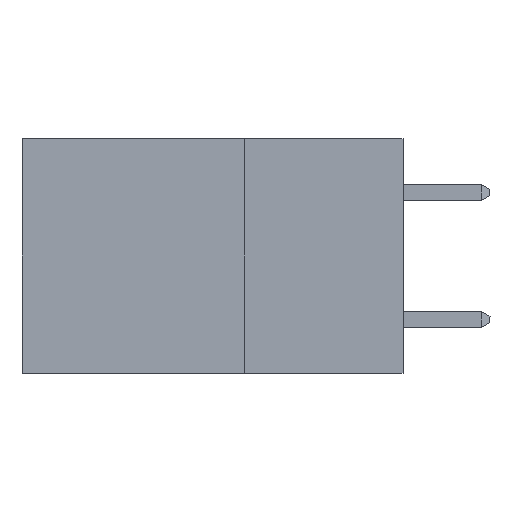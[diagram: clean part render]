
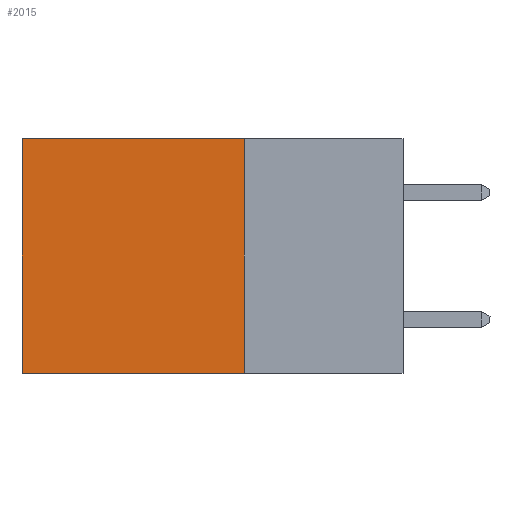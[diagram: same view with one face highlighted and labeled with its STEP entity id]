
A CAD part, left-side view. The second image highlights one B-rep face of the part: STEP entity #2015.
In plain terms, the highlighted planar face has unit normal (-1, 0, 0).
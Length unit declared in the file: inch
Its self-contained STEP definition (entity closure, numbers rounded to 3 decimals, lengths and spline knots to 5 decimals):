
#358 = VERTEX_POINT ( 'NONE', #6611 ) ;
#399 = AXIS2_PLACEMENT_3D ( 'NONE', #697, #4720, #6745 ) ;
#561 = VERTEX_POINT ( 'NONE', #2709 ) ;
#697 = CARTESIAN_POINT ( 'NONE',  ( 0.2875, 0.25, 0. ) ) ;
#1457 = LINE ( 'NONE', #3317, #11266 ) ;
#1633 = EDGE_CURVE ( 'NONE', #4223, #561, #1994, .T. ) ;
#1644 = PLANE ( 'NONE',  #399 ) ;
#1994 = LINE ( 'NONE', #8250, #9449 ) ;
#2015 = ADVANCED_FACE ( 'NONE', ( #6815 ), #1644, .F. ) ;
#2630 = DIRECTION ( 'NONE',  ( 0., 0., -1. ) ) ;
#2709 = CARTESIAN_POINT ( 'NONE',  ( 0.2875, 0.6, -0.37 ) ) ;
#2803 = CARTESIAN_POINT ( 'NONE',  ( 0.2875, 0.25, -0.37 ) ) ;
#2995 = EDGE_CURVE ( 'NONE', #3284, #358, #5194, .T. ) ;
#3284 = VERTEX_POINT ( 'NONE', #6817 ) ;
#3317 = CARTESIAN_POINT ( 'NONE',  ( 0.2875, 0.25, 0. ) ) ;
#3646 = LINE ( 'NONE', #8833, #11497 ) ;
#4223 = VERTEX_POINT ( 'NONE', #2803 ) ;
#4720 = DIRECTION ( 'NONE',  ( 1., 0., 0. ) ) ;
#5014 = ORIENTED_EDGE ( 'NONE', *, *, #5019, .T. ) ;
#5019 = EDGE_CURVE ( 'NONE', #358, #561, #3646, .T. ) ;
#5194 = LINE ( 'NONE', #6267, #9947 ) ;
#5873 = EDGE_CURVE ( 'NONE', #3284, #4223, #1457, .T. ) ;
#6267 = CARTESIAN_POINT ( 'NONE',  ( 0.2875, 0.25, 0. ) ) ;
#6611 = CARTESIAN_POINT ( 'NONE',  ( 0.2875, 0.6, 0. ) ) ;
#6745 = DIRECTION ( 'NONE',  ( 0., 0., -1. ) ) ;
#6815 = FACE_OUTER_BOUND ( 'NONE', #11611, .T. ) ;
#6817 = CARTESIAN_POINT ( 'NONE',  ( 0.2875, 0.25, 0. ) ) ;
#7578 = ORIENTED_EDGE ( 'NONE', *, *, #1633, .F. ) ;
#8250 = CARTESIAN_POINT ( 'NONE',  ( 0.2875, 0.25, -0.37 ) ) ;
#8833 = CARTESIAN_POINT ( 'NONE',  ( 0.2875, 0.6, 0. ) ) ;
#9449 = VECTOR ( 'NONE', #12331, 39.37008 ) ;
#9947 = VECTOR ( 'NONE', #11298, 39.37008 ) ;
#10048 = ORIENTED_EDGE ( 'NONE', *, *, #2995, .T. ) ;
#11266 = VECTOR ( 'NONE', #12665, 39.37008 ) ;
#11298 = DIRECTION ( 'NONE',  ( 0., 1., 0. ) ) ;
#11497 = VECTOR ( 'NONE', #2630, 39.37008 ) ;
#11611 = EDGE_LOOP ( 'NONE', ( #5014, #7578, #11807, #10048 ) ) ;
#11807 = ORIENTED_EDGE ( 'NONE', *, *, #5873, .F. ) ;
#12331 = DIRECTION ( 'NONE',  ( 0., 1., 0. ) ) ;
#12665 = DIRECTION ( 'NONE',  ( 0., 0., -1. ) ) ;
